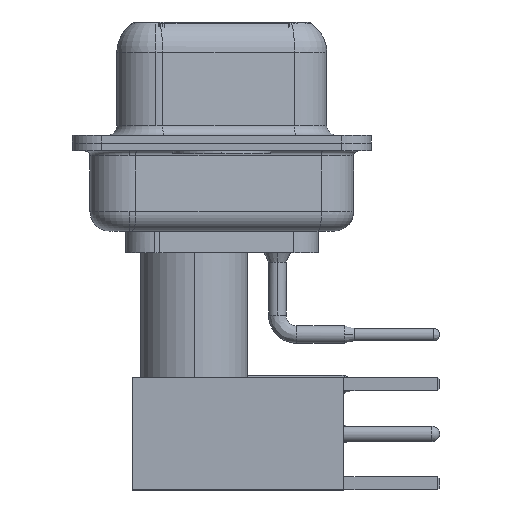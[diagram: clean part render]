
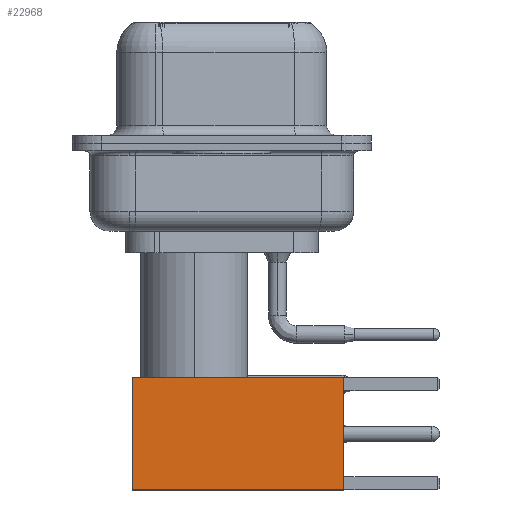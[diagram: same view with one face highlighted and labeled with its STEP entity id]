
A CAD part, left-side view. The second image highlights one B-rep face of the part: STEP entity #22968.
In plain terms, the highlighted face is planar.
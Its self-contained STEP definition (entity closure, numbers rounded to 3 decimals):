
#298 = DIRECTION ( 'NONE',  ( -1., 0., 0. ) ) ;
#1534 = LINE ( 'NONE', #4299, #20694 ) ;
#1601 = EDGE_CURVE ( 'NONE', #10201, #20093, #18278, .T. ) ;
#3064 = CARTESIAN_POINT ( 'NONE',  ( 0., 2.875, 0. ) ) ;
#4299 = CARTESIAN_POINT ( 'NONE',  ( 0., 2.875, 10.82 ) ) ;
#5829 = CARTESIAN_POINT ( 'NONE',  ( -2.875, 2.875, 0. ) ) ;
#7378 = VERTEX_POINT ( 'NONE', #10471 ) ;
#7582 = AXIS2_PLACEMENT_3D ( 'NONE', #12119, #27998, #30104 ) ;
#8066 = CARTESIAN_POINT ( 'NONE',  ( -2.875, 2.875, 10.82 ) ) ;
#8665 = EDGE_CURVE ( 'NONE', #31890, #20093, #23268, .T. ) ;
#8962 = EDGE_LOOP ( 'NONE', ( #21852, #16803, #21375, #30308 ) ) ;
#10201 = VERTEX_POINT ( 'NONE', #8066 ) ;
#10471 = CARTESIAN_POINT ( 'NONE',  ( 2.875, 2.875, 10.82 ) ) ;
#10566 = CARTESIAN_POINT ( 'NONE',  ( -2.875, 2.875, 0. ) ) ;
#11008 = DIRECTION ( 'NONE',  ( 0., 0., -1. ) ) ;
#11711 = VECTOR ( 'NONE', #298, 1000. ) ;
#11810 = VECTOR ( 'NONE', #11008, 1000. ) ;
#12072 = DIRECTION ( 'NONE',  ( -1., 0., 0. ) ) ;
#12119 = CARTESIAN_POINT ( 'NONE',  ( 2.875, 2.875, 0. ) ) ;
#12295 = FACE_OUTER_BOUND ( 'NONE', #8962, .T. ) ;
#12466 = PLANE ( 'NONE',  #7582 ) ;
#13078 = CARTESIAN_POINT ( 'NONE',  ( 2.875, 2.875, 0. ) ) ;
#13204 = VECTOR ( 'NONE', #15984, 1000. ) ;
#14354 = CARTESIAN_POINT ( 'NONE',  ( 2.875, 2.875, 0. ) ) ;
#15984 = DIRECTION ( 'NONE',  ( 0., 0., -1. ) ) ;
#16803 = ORIENTED_EDGE ( 'NONE', *, *, #8665, .T. ) ;
#18278 = LINE ( 'NONE', #5829, #11810 ) ;
#20093 = VERTEX_POINT ( 'NONE', #10566 ) ;
#20694 = VECTOR ( 'NONE', #12072, 1000. ) ;
#20827 = EDGE_CURVE ( 'NONE', #7378, #10201, #1534, .T. ) ;
#21328 = LINE ( 'NONE', #13078, #13204 ) ;
#21375 = ORIENTED_EDGE ( 'NONE', *, *, #1601, .F. ) ;
#21852 = ORIENTED_EDGE ( 'NONE', *, *, #32682, .T. ) ;
#22968 = ADVANCED_FACE ( 'NONE', ( #12295 ), #12466, .T. ) ;
#23268 = LINE ( 'NONE', #3064, #11711 ) ;
#27998 = DIRECTION ( 'NONE',  ( 0., 1., 0. ) ) ;
#30104 = DIRECTION ( 'NONE',  ( 0., 0., 1. ) ) ;
#30308 = ORIENTED_EDGE ( 'NONE', *, *, #20827, .F. ) ;
#31890 = VERTEX_POINT ( 'NONE', #14354 ) ;
#32682 = EDGE_CURVE ( 'NONE', #7378, #31890, #21328, .T. ) ;
